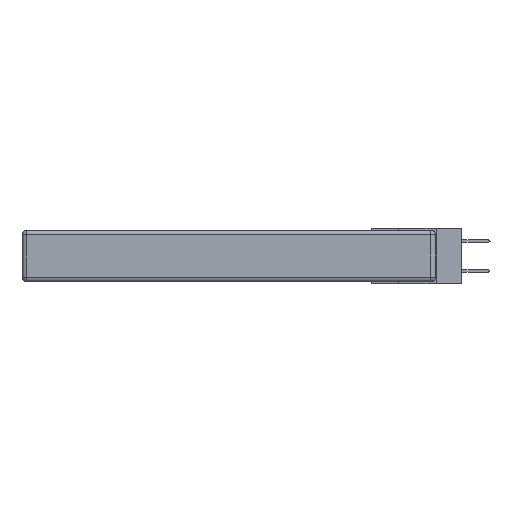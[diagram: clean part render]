
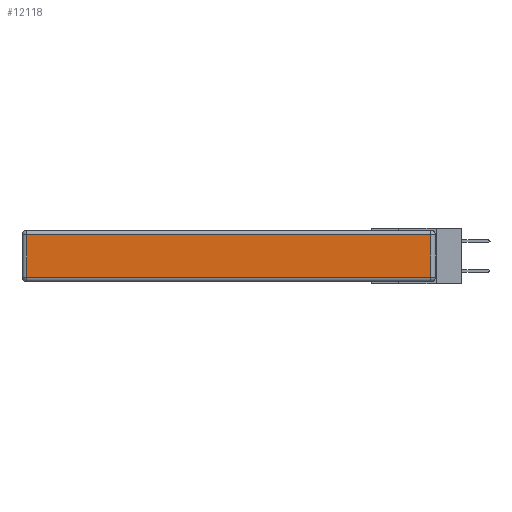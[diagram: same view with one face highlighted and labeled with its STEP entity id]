
A CAD part, left-side view. The second image highlights one B-rep face of the part: STEP entity #12118.
In plain terms, the highlighted planar face has unit normal (-1, 0, 0).
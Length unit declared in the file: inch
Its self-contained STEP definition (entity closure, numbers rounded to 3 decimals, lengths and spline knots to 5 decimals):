
#1745 = DIRECTION ( 'NONE',  ( 0., 1., 0. ) ) ;
#2986 = VERTEX_POINT ( 'NONE', #24913 ) ;
#3571 = VECTOR ( 'NONE', #25743, 39.37008 ) ;
#3903 = VECTOR ( 'NONE', #13615, 39.37008 ) ;
#4634 = LINE ( 'NONE', #25070, #3903 ) ;
#7358 = LINE ( 'NONE', #7777, #10177 ) ;
#7777 = CARTESIAN_POINT ( 'NONE',  ( 0., 0., -0.313 ) ) ;
#8126 = EDGE_CURVE ( 'NONE', #2986, #21353, #4634, .T. ) ;
#8740 = VECTOR ( 'NONE', #1745, 39.37008 ) ;
#9298 = CARTESIAN_POINT ( 'NONE',  ( 0., 2.72, -0.313 ) ) ;
#10177 = VECTOR ( 'NONE', #10221, 39.37008 ) ;
#10221 = DIRECTION ( 'NONE',  ( 0., -1., 0. ) ) ;
#10343 = ORIENTED_EDGE ( 'NONE', *, *, #8126, .T. ) ;
#11516 = CARTESIAN_POINT ( 'NONE',  ( 0., 2.72, -0.03 ) ) ;
#12118 = ADVANCED_FACE ( 'NONE', ( #26545 ), #17542, .T. ) ;
#12661 = LINE ( 'NONE', #23492, #3571 ) ;
#13084 = DIRECTION ( 'NONE',  ( -1., 0., 0. ) ) ;
#13615 = DIRECTION ( 'NONE',  ( 0., 0., 1. ) ) ;
#14871 = ORIENTED_EDGE ( 'NONE', *, *, #15817, .T. ) ;
#15067 = DIRECTION ( 'NONE',  ( 0., 0., 1. ) ) ;
#15817 = EDGE_CURVE ( 'NONE', #24008, #16947, #12661, .T. ) ;
#16355 = EDGE_CURVE ( 'NONE', #16947, #2986, #7358, .T. ) ;
#16497 = EDGE_CURVE ( 'NONE', #21353, #24008, #18605, .T. ) ;
#16947 = VERTEX_POINT ( 'NONE', #9298 ) ;
#17542 = PLANE ( 'NONE',  #18531 ) ;
#18531 = AXIS2_PLACEMENT_3D ( 'NONE', #19809, #13084, #15067 ) ;
#18605 = LINE ( 'NONE', #26916, #8740 ) ;
#19748 = ORIENTED_EDGE ( 'NONE', *, *, #16497, .T. ) ;
#19809 = CARTESIAN_POINT ( 'NONE',  ( 0., 0., -0.343 ) ) ;
#20227 = CARTESIAN_POINT ( 'NONE',  ( 0., 0.03, -0.03 ) ) ;
#21353 = VERTEX_POINT ( 'NONE', #20227 ) ;
#23492 = CARTESIAN_POINT ( 'NONE',  ( 0., 2.72, -0.343 ) ) ;
#24008 = VERTEX_POINT ( 'NONE', #11516 ) ;
#24913 = CARTESIAN_POINT ( 'NONE',  ( 0., 0.03, -0.313 ) ) ;
#25020 = ORIENTED_EDGE ( 'NONE', *, *, #16355, .T. ) ;
#25070 = CARTESIAN_POINT ( 'NONE',  ( 0., 0.03, -0.343 ) ) ;
#25743 = DIRECTION ( 'NONE',  ( 0., 0., -1. ) ) ;
#26545 = FACE_OUTER_BOUND ( 'NONE', #29114, .T. ) ;
#26916 = CARTESIAN_POINT ( 'NONE',  ( 0., 2.75, -0.03 ) ) ;
#29114 = EDGE_LOOP ( 'NONE', ( #25020, #10343, #19748, #14871 ) ) ;
